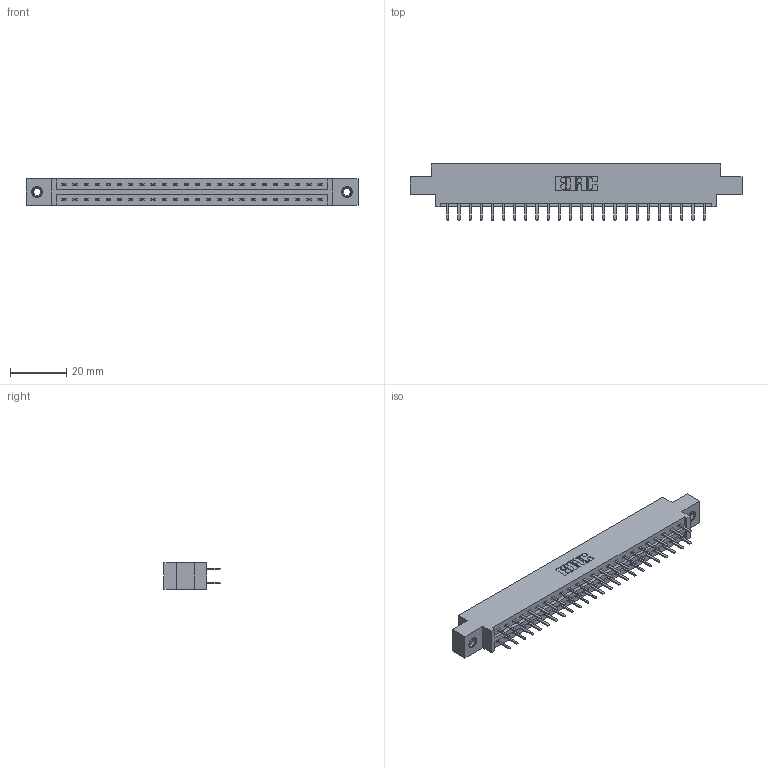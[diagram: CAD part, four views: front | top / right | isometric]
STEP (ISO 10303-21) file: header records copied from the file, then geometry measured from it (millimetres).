
FILE_DESCRIPTION (( 'STEP AP203' ), '1' );
FILE_NAME ('337-048-520-807.STEP', '2019-10-11T15:09:55', ( '' ), ( '' ), 'SwSTEP 2.0', 'SolidWorks 2016', '' );
FILE_SCHEMA (( 'CONFIG_CONTROL_DESIGN' ));
Length unit declared in the file: inch
Products named in the file (4): 337-048-520-807; 345-250-001_345-250-005-103; 345-292-001_345-293-120; 337 Part_0.170 Offset - 0.156 Dia-TI
Assembly tree (51 placements, depth 2):
  337-048-520-807
    337 Part_0.170 Offset - 0.156 Dia-TI
    345-292-001_345-293-120  x48
    345-250-001_345-250-005-103  x2
Bounding box: 118.11 x 20.02 x 9.4 mm (x, y, z)
Volume: 12055.6 mm3; surface area: 13537.7 mm2
Topology: 51 solids, 51 shells, 2962 faces, 8571 edges, 5578 vertices
Faces by surface type: plane 2026, cylinder 920, cone 12, torus 4
Entity records: 22368 total; most frequent: CARTESIAN_POINT 3777, ORIENTED_EDGE 3694, DIRECTION 3265, EDGE_CURVE 1847, LINE 1695, VECTOR 1695, VERTEX_POINT 1224, AXIS2_PLACEMENT_3D 785
